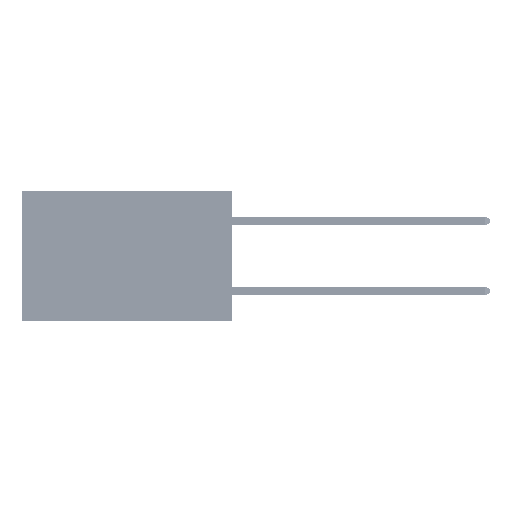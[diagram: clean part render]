
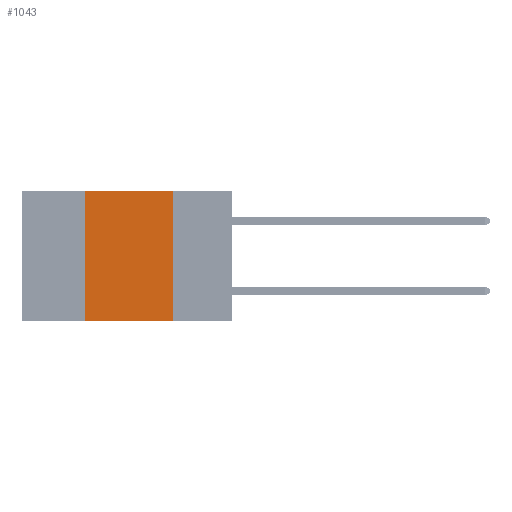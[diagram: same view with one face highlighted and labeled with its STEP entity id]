
A CAD part, left-side view. The second image highlights one B-rep face of the part: STEP entity #1043.
In plain terms, the highlighted planar face has unit normal (-1, 0, 0).
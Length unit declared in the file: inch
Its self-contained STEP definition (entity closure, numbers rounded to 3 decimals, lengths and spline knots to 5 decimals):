
#961 = AXIS2_PLACEMENT_3D ( 'NONE', #15977, #8731, #23978 ) ;
#1043 = ADVANCED_FACE ( 'NONE', ( #41885 ), #4641, .F. ) ;
#1737 = EDGE_CURVE ( 'NONE', #49902, #21402, #27032, .T. ) ;
#2277 = EDGE_CURVE ( 'NONE', #32211, #28198, #4938, .T. ) ;
#3409 = ORIENTED_EDGE ( 'NONE', *, *, #45487, .T. ) ;
#4641 = PLANE ( 'NONE',  #961 ) ;
#4938 = LINE ( 'NONE', #45904, #16591 ) ;
#6799 = DIRECTION ( 'NONE',  ( 0., 0., 1. ) ) ;
#7234 = DIRECTION ( 'NONE',  ( 0., 0., -1. ) ) ;
#8731 = DIRECTION ( 'NONE',  ( 1., 0., 0. ) ) ;
#11430 = EDGE_LOOP ( 'NONE', ( #33647, #37649, #40380, #3409 ) ) ;
#11487 = VECTOR ( 'NONE', #31973, 39.37008 ) ;
#15977 = CARTESIAN_POINT ( 'NONE',  ( 0., 0.6, 0. ) ) ;
#16591 = VECTOR ( 'NONE', #7234, 39.37008 ) ;
#18285 = CARTESIAN_POINT ( 'NONE',  ( 0., 0.6, -0.37 ) ) ;
#21402 = VERTEX_POINT ( 'NONE', #28134 ) ;
#21599 = CARTESIAN_POINT ( 'NONE',  ( 0., 0.42, -0.37 ) ) ;
#22088 = CARTESIAN_POINT ( 'NONE',  ( 0., 0.17, 0. ) ) ;
#23749 = CARTESIAN_POINT ( 'NONE',  ( 0., 0.6, 0. ) ) ;
#23978 = DIRECTION ( 'NONE',  ( 0., 0., -1. ) ) ;
#27032 = LINE ( 'NONE', #45792, #28882 ) ;
#28134 = CARTESIAN_POINT ( 'NONE',  ( 0., 0.42, 0. ) ) ;
#28198 = VERTEX_POINT ( 'NONE', #41355 ) ;
#28882 = VECTOR ( 'NONE', #6799, 39.37008 ) ;
#31973 = DIRECTION ( 'NONE',  ( 0., -1., 0. ) ) ;
#32211 = VERTEX_POINT ( 'NONE', #22088 ) ;
#33647 = ORIENTED_EDGE ( 'NONE', *, *, #2277, .F. ) ;
#35769 = LINE ( 'NONE', #18285, #38203 ) ;
#37649 = ORIENTED_EDGE ( 'NONE', *, *, #43389, .F. ) ;
#38203 = VECTOR ( 'NONE', #42024, 39.37008 ) ;
#40246 = LINE ( 'NONE', #23749, #11487 ) ;
#40380 = ORIENTED_EDGE ( 'NONE', *, *, #1737, .F. ) ;
#41355 = CARTESIAN_POINT ( 'NONE',  ( 0., 0.17, -0.37 ) ) ;
#41885 = FACE_OUTER_BOUND ( 'NONE', #11430, .T. ) ;
#42024 = DIRECTION ( 'NONE',  ( 0., -1., 0. ) ) ;
#43389 = EDGE_CURVE ( 'NONE', #21402, #32211, #40246, .T. ) ;
#45487 = EDGE_CURVE ( 'NONE', #49902, #28198, #35769, .T. ) ;
#45792 = CARTESIAN_POINT ( 'NONE',  ( 0., 0.42, 0. ) ) ;
#45904 = CARTESIAN_POINT ( 'NONE',  ( 0., 0.17, 0. ) ) ;
#49902 = VERTEX_POINT ( 'NONE', #21599 ) ;
